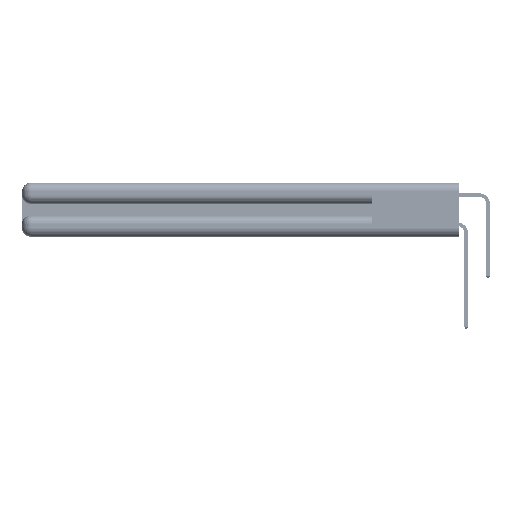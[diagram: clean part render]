
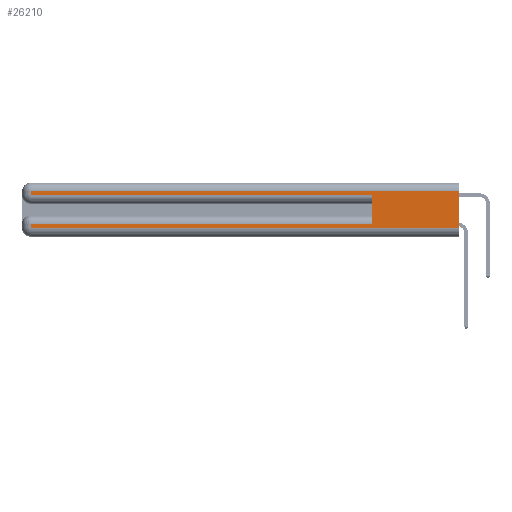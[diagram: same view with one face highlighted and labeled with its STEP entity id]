
A CAD part, left-side view. The second image highlights one B-rep face of the part: STEP entity #26210.
In plain terms, the highlighted planar face has unit normal (-1, 0, 0).
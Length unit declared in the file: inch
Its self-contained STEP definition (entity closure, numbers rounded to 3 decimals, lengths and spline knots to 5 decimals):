
#95 = EDGE_CURVE ( 'NONE', #28711, #23117, #38701, .T. ) ;
#499 = DIRECTION ( 'NONE',  ( 0., 0., -1. ) ) ;
#2017 = VERTEX_POINT ( 'NONE', #53389 ) ;
#2249 = EDGE_CURVE ( 'NONE', #2017, #28711, #16498, .T. ) ;
#3638 = FACE_OUTER_BOUND ( 'NONE', #50799, .T. ) ;
#4196 = CARTESIAN_POINT ( 'NONE',  ( 0., 2.94, 0.37 ) ) ;
#6121 = ORIENTED_EDGE ( 'NONE', *, *, #39343, .T. ) ;
#7436 = EDGE_CURVE ( 'NONE', #2017, #52003, #9189, .T. ) ;
#8692 = PLANE ( 'NONE',  #27050 ) ;
#9150 = DIRECTION ( 'NONE',  ( 0., -1., 0. ) ) ;
#9189 = LINE ( 'NONE', #44017, #41723 ) ;
#10487 = ORIENTED_EDGE ( 'NONE', *, *, #43890, .F. ) ;
#12310 = DIRECTION ( 'NONE',  ( 0., 1., 0. ) ) ;
#12320 = CARTESIAN_POINT ( 'NONE',  ( 0., 2.94, 0.31 ) ) ;
#12606 = ORIENTED_EDGE ( 'NONE', *, *, #13224, .T. ) ;
#12736 = DIRECTION ( 'NONE',  ( 0., 0., -1. ) ) ;
#13224 = EDGE_CURVE ( 'NONE', #44282, #16493, #35167, .T. ) ;
#14500 = EDGE_CURVE ( 'NONE', #16493, #52003, #30198, .T. ) ;
#15426 = CARTESIAN_POINT ( 'NONE',  ( 0., 2.94, 0.06 ) ) ;
#15891 = VECTOR ( 'NONE', #16852, 39.37008 ) ;
#16493 = VERTEX_POINT ( 'NONE', #56823 ) ;
#16498 = LINE ( 'NONE', #34425, #22037 ) ;
#16827 = DIRECTION ( 'NONE',  ( 0., 1., 0. ) ) ;
#16852 = DIRECTION ( 'NONE',  ( 0., 0., -1. ) ) ;
#17456 = ORIENTED_EDGE ( 'NONE', *, *, #2249, .T. ) ;
#17995 = DIRECTION ( 'NONE',  ( 1., 0., 0. ) ) ;
#21030 = CARTESIAN_POINT ( 'NONE',  ( 0., 0., 0.285 ) ) ;
#21622 = CARTESIAN_POINT ( 'NONE',  ( 0., 0., 0.31 ) ) ;
#22037 = VECTOR ( 'NONE', #16827, 39.37008 ) ;
#23117 = VERTEX_POINT ( 'NONE', #15426 ) ;
#25348 = CARTESIAN_POINT ( 'NONE',  ( 0., 2.94, 0.085 ) ) ;
#26210 = ADVANCED_FACE ( 'NONE', ( #3638 ), #8692, .F. ) ;
#27050 = AXIS2_PLACEMENT_3D ( 'NONE', #52801, #17995, #499 ) ;
#27419 = LINE ( 'NONE', #49379, #51595 ) ;
#28711 = VERTEX_POINT ( 'NONE', #25348 ) ;
#30080 = VERTEX_POINT ( 'NONE', #21622 ) ;
#30198 = LINE ( 'NONE', #21030, #46748 ) ;
#30426 = CARTESIAN_POINT ( 'NONE',  ( 0., 2.94, 0.37 ) ) ;
#30573 = VECTOR ( 'NONE', #44079, 39.37008 ) ;
#31628 = CARTESIAN_POINT ( 'NONE',  ( 0., 0.6, 0.285 ) ) ;
#34425 = CARTESIAN_POINT ( 'NONE',  ( 0., 0., 0.085 ) ) ;
#34647 = ORIENTED_EDGE ( 'NONE', *, *, #7436, .F. ) ;
#35130 = EDGE_CURVE ( 'NONE', #23117, #48074, #27419, .T. ) ;
#35167 = LINE ( 'NONE', #4196, #48297 ) ;
#37482 = LINE ( 'NONE', #38446, #40861 ) ;
#38446 = CARTESIAN_POINT ( 'NONE',  ( 0., 0., 0.31 ) ) ;
#38701 = LINE ( 'NONE', #30426, #15891 ) ;
#39343 = EDGE_CURVE ( 'NONE', #30080, #44282, #37482, .T. ) ;
#40347 = DIRECTION ( 'NONE',  ( 0., 0., 1. ) ) ;
#40861 = VECTOR ( 'NONE', #12310, 39.37008 ) ;
#41723 = VECTOR ( 'NONE', #40347, 39.37008 ) ;
#42893 = DIRECTION ( 'NONE',  ( 0., -1., 0. ) ) ;
#43603 = CARTESIAN_POINT ( 'NONE',  ( 0., 0., 0.06 ) ) ;
#43890 = EDGE_CURVE ( 'NONE', #30080, #48074, #47838, .T. ) ;
#44017 = CARTESIAN_POINT ( 'NONE',  ( 0., 0.6, 0.145 ) ) ;
#44079 = DIRECTION ( 'NONE',  ( 0., 0., -1. ) ) ;
#44120 = ORIENTED_EDGE ( 'NONE', *, *, #95, .T. ) ;
#44274 = CARTESIAN_POINT ( 'NONE',  ( 0., 0., 0.37 ) ) ;
#44282 = VERTEX_POINT ( 'NONE', #12320 ) ;
#45042 = ORIENTED_EDGE ( 'NONE', *, *, #35130, .T. ) ;
#46748 = VECTOR ( 'NONE', #42893, 39.37008 ) ;
#47838 = LINE ( 'NONE', #44274, #30573 ) ;
#48074 = VERTEX_POINT ( 'NONE', #43603 ) ;
#48297 = VECTOR ( 'NONE', #12736, 39.37008 ) ;
#49379 = CARTESIAN_POINT ( 'NONE',  ( 0., 0., 0.06 ) ) ;
#50799 = EDGE_LOOP ( 'NONE', ( #10487, #6121, #12606, #55827, #34647, #17456, #44120, #45042 ) ) ;
#51595 = VECTOR ( 'NONE', #9150, 39.37008 ) ;
#52003 = VERTEX_POINT ( 'NONE', #31628 ) ;
#52801 = CARTESIAN_POINT ( 'NONE',  ( 0., 0., 0.37 ) ) ;
#53389 = CARTESIAN_POINT ( 'NONE',  ( 0., 0.6, 0.085 ) ) ;
#55827 = ORIENTED_EDGE ( 'NONE', *, *, #14500, .T. ) ;
#56823 = CARTESIAN_POINT ( 'NONE',  ( 0., 2.94, 0.285 ) ) ;
